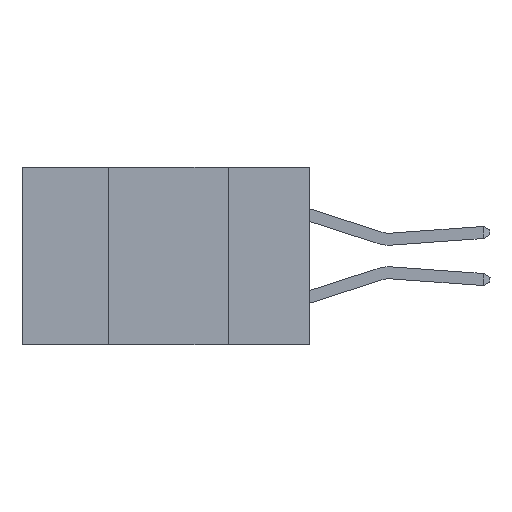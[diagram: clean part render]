
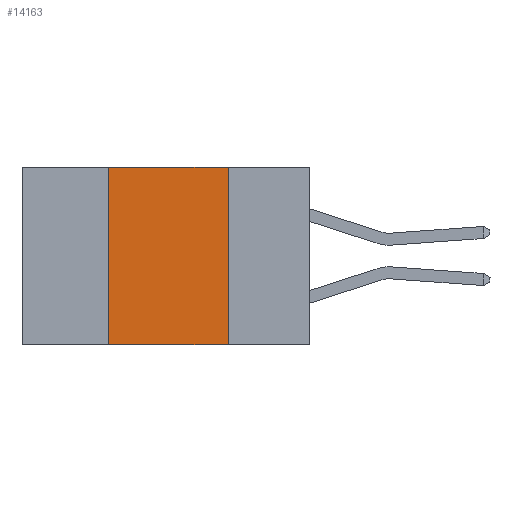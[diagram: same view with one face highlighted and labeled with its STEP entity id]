
A CAD part, left-side view. The second image highlights one B-rep face of the part: STEP entity #14163.
In plain terms, the highlighted planar face has unit normal (-1, 0, 0).
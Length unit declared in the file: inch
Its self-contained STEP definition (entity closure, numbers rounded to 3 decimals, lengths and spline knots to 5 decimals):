
#462 = VECTOR ( 'NONE', #3451, 39.37008 ) ;
#792 = CARTESIAN_POINT ( 'NONE',  ( 0., 0.42, 0. ) ) ;
#1018 = CARTESIAN_POINT ( 'NONE',  ( 0., 0.17, 0. ) ) ;
#2209 = CARTESIAN_POINT ( 'NONE',  ( 0., 0.17, 0. ) ) ;
#2396 = CARTESIAN_POINT ( 'NONE',  ( 0., 0.42, -0.37 ) ) ;
#2938 = VECTOR ( 'NONE', #8726, 39.37008 ) ;
#3451 = DIRECTION ( 'NONE',  ( 0., 0., -1. ) ) ;
#3504 = AXIS2_PLACEMENT_3D ( 'NONE', #4331, #14526, #13290 ) ;
#3743 = LINE ( 'NONE', #12682, #7496 ) ;
#3784 = LINE ( 'NONE', #5947, #9456 ) ;
#4021 = EDGE_LOOP ( 'NONE', ( #13735, #13069, #13394, #4940 ) ) ;
#4331 = CARTESIAN_POINT ( 'NONE',  ( 0., 0.6, 0. ) ) ;
#4471 = EDGE_CURVE ( 'NONE', #5418, #10729, #3784, .T. ) ;
#4940 = ORIENTED_EDGE ( 'NONE', *, *, #4471, .T. ) ;
#5418 = VERTEX_POINT ( 'NONE', #2396 ) ;
#5656 = VERTEX_POINT ( 'NONE', #1018 ) ;
#5947 = CARTESIAN_POINT ( 'NONE',  ( 0., 0.6, -0.37 ) ) ;
#6047 = CARTESIAN_POINT ( 'NONE',  ( 0., 0.42, 0. ) ) ;
#7496 = VECTOR ( 'NONE', #8099, 39.37008 ) ;
#8099 = DIRECTION ( 'NONE',  ( 0., -1., 0. ) ) ;
#8120 = CARTESIAN_POINT ( 'NONE',  ( 0., 0.17, -0.37 ) ) ;
#8726 = DIRECTION ( 'NONE',  ( 0., 0., 1. ) ) ;
#9456 = VECTOR ( 'NONE', #11600, 39.37008 ) ;
#9646 = LINE ( 'NONE', #2209, #462 ) ;
#10385 = FACE_OUTER_BOUND ( 'NONE', #4021, .T. ) ;
#10729 = VERTEX_POINT ( 'NONE', #8120 ) ;
#10975 = PLANE ( 'NONE',  #3504 ) ;
#11490 = EDGE_CURVE ( 'NONE', #5418, #12814, #12644, .T. ) ;
#11600 = DIRECTION ( 'NONE',  ( 0., -1., 0. ) ) ;
#12091 = EDGE_CURVE ( 'NONE', #5656, #10729, #9646, .T. ) ;
#12644 = LINE ( 'NONE', #792, #2938 ) ;
#12682 = CARTESIAN_POINT ( 'NONE',  ( 0., 0.6, 0. ) ) ;
#12814 = VERTEX_POINT ( 'NONE', #6047 ) ;
#13069 = ORIENTED_EDGE ( 'NONE', *, *, #13862, .F. ) ;
#13290 = DIRECTION ( 'NONE',  ( 0., 0., -1. ) ) ;
#13394 = ORIENTED_EDGE ( 'NONE', *, *, #11490, .F. ) ;
#13735 = ORIENTED_EDGE ( 'NONE', *, *, #12091, .F. ) ;
#13862 = EDGE_CURVE ( 'NONE', #12814, #5656, #3743, .T. ) ;
#14163 = ADVANCED_FACE ( 'NONE', ( #10385 ), #10975, .F. ) ;
#14526 = DIRECTION ( 'NONE',  ( 1., 0., 0. ) ) ;
